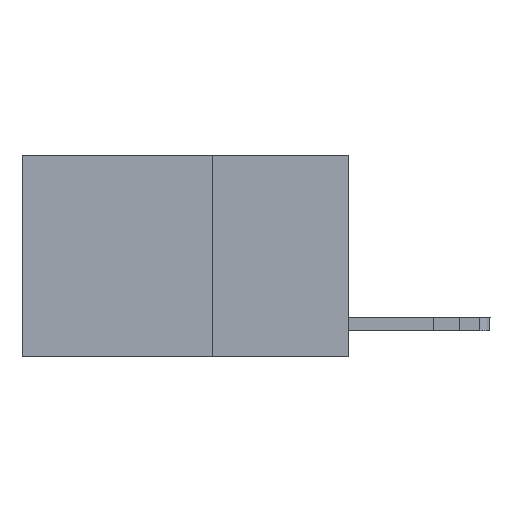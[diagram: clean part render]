
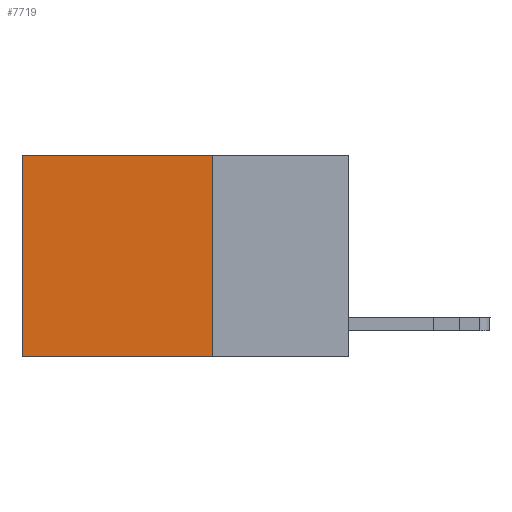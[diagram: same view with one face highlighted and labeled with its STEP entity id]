
A CAD part, left-side view. The second image highlights one B-rep face of the part: STEP entity #7719.
In plain terms, the highlighted planar face has unit normal (-1, 0, 0).
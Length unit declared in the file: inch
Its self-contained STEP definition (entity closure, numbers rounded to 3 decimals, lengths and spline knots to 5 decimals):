
#165 = CARTESIAN_POINT ( 'NONE',  ( 0.2625, 0.6, 0. ) ) ;
#311 = DIRECTION ( 'NONE',  ( 0., 0., -1. ) ) ;
#533 = CARTESIAN_POINT ( 'NONE',  ( 0.2625, 0.25, -0.37 ) ) ;
#2147 = FACE_OUTER_BOUND ( 'NONE', #3039, .T. ) ;
#2210 = ORIENTED_EDGE ( 'NONE', *, *, #14081, .T. ) ;
#2564 = VECTOR ( 'NONE', #311, 39.37008 ) ;
#3039 = EDGE_LOOP ( 'NONE', ( #7012, #4076, #12970, #2210 ) ) ;
#3889 = DIRECTION ( 'NONE',  ( 0., 1., 0. ) ) ;
#4076 = ORIENTED_EDGE ( 'NONE', *, *, #4829, .F. ) ;
#4215 = CARTESIAN_POINT ( 'NONE',  ( 0.2625, 0.25, -0.37 ) ) ;
#4435 = CARTESIAN_POINT ( 'NONE',  ( 0.2625, 0.25, 0. ) ) ;
#4448 = VECTOR ( 'NONE', #5075, 39.37008 ) ;
#4790 = VERTEX_POINT ( 'NONE', #10569 ) ;
#4829 = EDGE_CURVE ( 'NONE', #10137, #4790, #6150, .T. ) ;
#5075 = DIRECTION ( 'NONE',  ( 0., 0., -1. ) ) ;
#6150 = LINE ( 'NONE', #533, #13941 ) ;
#6151 = VERTEX_POINT ( 'NONE', #7148 ) ;
#6453 = EDGE_CURVE ( 'NONE', #6151, #10137, #7181, .T. ) ;
#6778 = CARTESIAN_POINT ( 'NONE',  ( 0.2625, 0.6, 0. ) ) ;
#7012 = ORIENTED_EDGE ( 'NONE', *, *, #10286, .T. ) ;
#7095 = VECTOR ( 'NONE', #10138, 39.37008 ) ;
#7148 = CARTESIAN_POINT ( 'NONE',  ( 0.2625, 0.25, 0. ) ) ;
#7181 = LINE ( 'NONE', #12606, #4448 ) ;
#7658 = PLANE ( 'NONE',  #9969 ) ;
#7719 = ADVANCED_FACE ( 'NONE', ( #2147 ), #7658, .F. ) ;
#7720 = DIRECTION ( 'NONE',  ( 1., 0., 0. ) ) ;
#8692 = VERTEX_POINT ( 'NONE', #6778 ) ;
#9045 = LINE ( 'NONE', #4435, #7095 ) ;
#9969 = AXIS2_PLACEMENT_3D ( 'NONE', #12111, #7720, #12187 ) ;
#10137 = VERTEX_POINT ( 'NONE', #4215 ) ;
#10138 = DIRECTION ( 'NONE',  ( 0., 1., 0. ) ) ;
#10286 = EDGE_CURVE ( 'NONE', #8692, #4790, #10406, .T. ) ;
#10406 = LINE ( 'NONE', #165, #2564 ) ;
#10569 = CARTESIAN_POINT ( 'NONE',  ( 0.2625, 0.6, -0.37 ) ) ;
#12111 = CARTESIAN_POINT ( 'NONE',  ( 0.2625, 0.25, 0. ) ) ;
#12187 = DIRECTION ( 'NONE',  ( 0., 0., -1. ) ) ;
#12606 = CARTESIAN_POINT ( 'NONE',  ( 0.2625, 0.25, 0. ) ) ;
#12970 = ORIENTED_EDGE ( 'NONE', *, *, #6453, .F. ) ;
#13941 = VECTOR ( 'NONE', #3889, 39.37008 ) ;
#14081 = EDGE_CURVE ( 'NONE', #6151, #8692, #9045, .T. ) ;
